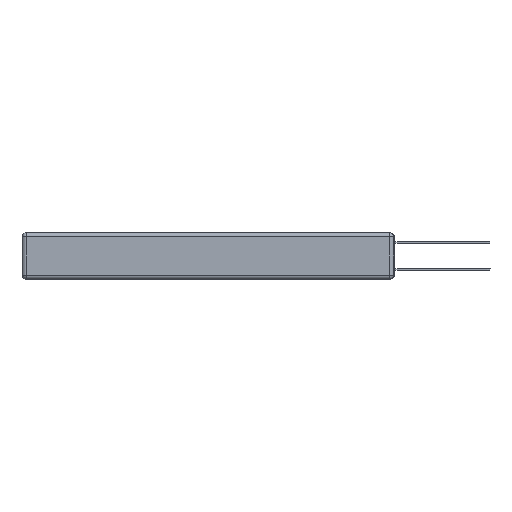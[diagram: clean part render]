
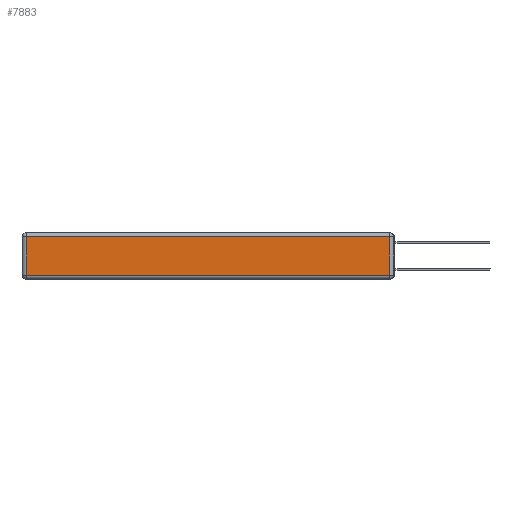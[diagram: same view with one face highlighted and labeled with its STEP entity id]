
A CAD part, left-side view. The second image highlights one B-rep face of the part: STEP entity #7883.
In plain terms, the highlighted planar face has unit normal (-1, 0, 0).
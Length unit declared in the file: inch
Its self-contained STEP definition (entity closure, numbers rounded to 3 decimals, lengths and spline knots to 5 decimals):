
#72 = ORIENTED_EDGE ( 'NONE', *, *, #2967, .T. ) ;
#259 = DIRECTION ( 'NONE',  ( -1., 0., 0. ) ) ;
#341 = FACE_OUTER_BOUND ( 'NONE', #13659, .T. ) ;
#492 = CARTESIAN_POINT ( 'NONE',  ( 0., 0., -0.313 ) ) ;
#1447 = EDGE_CURVE ( 'NONE', #15403, #2533, #3895, .T. ) ;
#2313 = VECTOR ( 'NONE', #15545, 39.37008 ) ;
#2533 = VERTEX_POINT ( 'NONE', #15188 ) ;
#2695 = AXIS2_PLACEMENT_3D ( 'NONE', #7906, #259, #6655 ) ;
#2909 = DIRECTION ( 'NONE',  ( 0., 1., 0. ) ) ;
#2967 = EDGE_CURVE ( 'NONE', #16246, #15403, #14028, .T. ) ;
#3846 = CARTESIAN_POINT ( 'NONE',  ( 0., 2.72, -0.343 ) ) ;
#3895 = LINE ( 'NONE', #492, #2313 ) ;
#6013 = ORIENTED_EDGE ( 'NONE', *, *, #1447, .T. ) ;
#6655 = DIRECTION ( 'NONE',  ( 0., 0., 1. ) ) ;
#7770 = VECTOR ( 'NONE', #11889, 39.37008 ) ;
#7883 = ADVANCED_FACE ( 'NONE', ( #341 ), #13107, .T. ) ;
#7906 = CARTESIAN_POINT ( 'NONE',  ( 0., 0., -0.343 ) ) ;
#7972 = CARTESIAN_POINT ( 'NONE',  ( 0., 2.75, -0.03 ) ) ;
#8521 = CARTESIAN_POINT ( 'NONE',  ( 0., 2.72, -0.03 ) ) ;
#8693 = ORIENTED_EDGE ( 'NONE', *, *, #9608, .T. ) ;
#9245 = EDGE_CURVE ( 'NONE', #2533, #13272, #10719, .T. ) ;
#9608 = EDGE_CURVE ( 'NONE', #13272, #16246, #10372, .T. ) ;
#10161 = DIRECTION ( 'NONE',  ( 0., 0., -1. ) ) ;
#10372 = LINE ( 'NONE', #7972, #11712 ) ;
#10719 = LINE ( 'NONE', #15817, #7770 ) ;
#11110 = CARTESIAN_POINT ( 'NONE',  ( 0., 0.03, -0.03 ) ) ;
#11712 = VECTOR ( 'NONE', #2909, 39.37008 ) ;
#11889 = DIRECTION ( 'NONE',  ( 0., 0., 1. ) ) ;
#13107 = PLANE ( 'NONE',  #2695 ) ;
#13272 = VERTEX_POINT ( 'NONE', #11110 ) ;
#13535 = ORIENTED_EDGE ( 'NONE', *, *, #9245, .T. ) ;
#13659 = EDGE_LOOP ( 'NONE', ( #6013, #13535, #8693, #72 ) ) ;
#14028 = LINE ( 'NONE', #3846, #15185 ) ;
#15185 = VECTOR ( 'NONE', #10161, 39.37008 ) ;
#15188 = CARTESIAN_POINT ( 'NONE',  ( 0., 0.03, -0.313 ) ) ;
#15403 = VERTEX_POINT ( 'NONE', #15996 ) ;
#15545 = DIRECTION ( 'NONE',  ( 0., -1., 0. ) ) ;
#15817 = CARTESIAN_POINT ( 'NONE',  ( 0., 0.03, -0.343 ) ) ;
#15996 = CARTESIAN_POINT ( 'NONE',  ( 0., 2.72, -0.313 ) ) ;
#16246 = VERTEX_POINT ( 'NONE', #8521 ) ;
